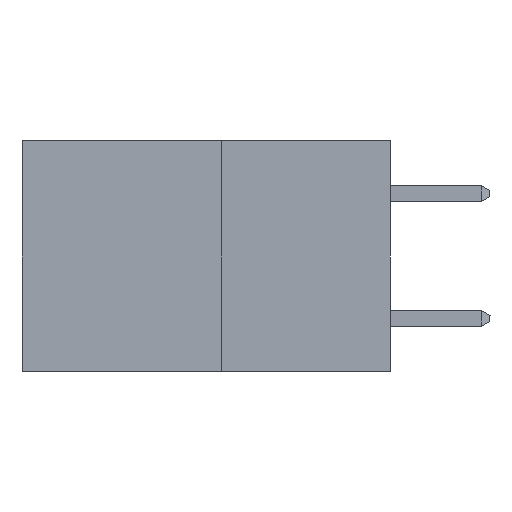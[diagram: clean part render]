
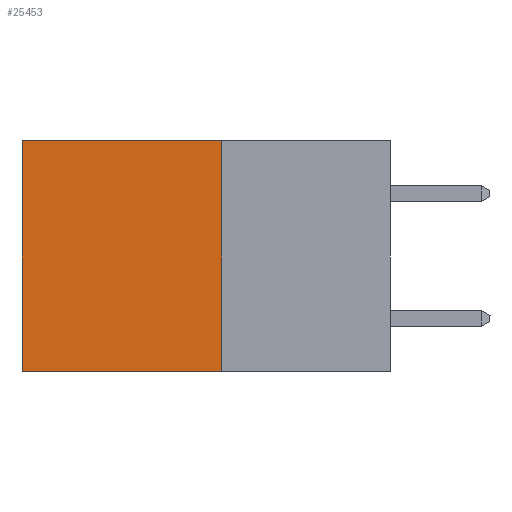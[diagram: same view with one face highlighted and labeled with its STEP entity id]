
A CAD part, left-side view. The second image highlights one B-rep face of the part: STEP entity #25453.
In plain terms, the highlighted planar face has unit normal (-1, 0, 0).
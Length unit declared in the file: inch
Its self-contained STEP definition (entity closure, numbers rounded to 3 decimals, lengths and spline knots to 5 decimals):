
#1934 = VERTEX_POINT ( 'NONE', #5317 ) ;
#2695 = DIRECTION ( 'NONE',  ( 0., 0., -1. ) ) ;
#4121 = EDGE_CURVE ( 'NONE', #22747, #12051, #9934, .T. ) ;
#4200 = ORIENTED_EDGE ( 'NONE', *, *, #4121, .T. ) ;
#5317 = CARTESIAN_POINT ( 'NONE',  ( 0.277, 0.27, 0. ) ) ;
#5670 = ORIENTED_EDGE ( 'NONE', *, *, #5870, .F. ) ;
#5870 = EDGE_CURVE ( 'NONE', #1934, #24438, #7227, .T. ) ;
#6961 = ORIENTED_EDGE ( 'NONE', *, *, #7106, .T. ) ;
#7106 = EDGE_CURVE ( 'NONE', #1934, #22747, #26792, .T. ) ;
#7227 = LINE ( 'NONE', #19819, #18918 ) ;
#7507 = CARTESIAN_POINT ( 'NONE',  ( 0.277, 0.27, -0.37 ) ) ;
#9934 = LINE ( 'NONE', #25748, #21575 ) ;
#10127 = CARTESIAN_POINT ( 'NONE',  ( 0.277, 0.59, -0.37 ) ) ;
#12051 = VERTEX_POINT ( 'NONE', #10127 ) ;
#12527 = EDGE_CURVE ( 'NONE', #24438, #12051, #24372, .T. ) ;
#14469 = PLANE ( 'NONE',  #19640 ) ;
#15068 = FACE_OUTER_BOUND ( 'NONE', #20076, .T. ) ;
#16757 = DIRECTION ( 'NONE',  ( 1., 0., 0. ) ) ;
#16781 = VECTOR ( 'NONE', #23798, 39.37008 ) ;
#18918 = VECTOR ( 'NONE', #29790, 39.37008 ) ;
#19404 = CARTESIAN_POINT ( 'NONE',  ( 0.277, 0.27, -0.37 ) ) ;
#19640 = AXIS2_PLACEMENT_3D ( 'NONE', #23631, #16757, #2695 ) ;
#19819 = CARTESIAN_POINT ( 'NONE',  ( 0.277, 0.27, -0.37 ) ) ;
#20076 = EDGE_LOOP ( 'NONE', ( #4200, #27887, #5670, #6961 ) ) ;
#20478 = CARTESIAN_POINT ( 'NONE',  ( 0.277, 0.59, 0. ) ) ;
#20780 = DIRECTION ( 'NONE',  ( 0., 1., 0. ) ) ;
#21409 = CARTESIAN_POINT ( 'NONE',  ( 0.277, 0.27, 0. ) ) ;
#21575 = VECTOR ( 'NONE', #24347, 39.37008 ) ;
#22747 = VERTEX_POINT ( 'NONE', #20478 ) ;
#23631 = CARTESIAN_POINT ( 'NONE',  ( 0.277, 0.27, -0.37 ) ) ;
#23798 = DIRECTION ( 'NONE',  ( 0., 1., 0. ) ) ;
#24347 = DIRECTION ( 'NONE',  ( 0., 0., -1. ) ) ;
#24372 = LINE ( 'NONE', #7507, #16781 ) ;
#24438 = VERTEX_POINT ( 'NONE', #19404 ) ;
#25369 = VECTOR ( 'NONE', #20780, 39.37008 ) ;
#25453 = ADVANCED_FACE ( 'NONE', ( #15068 ), #14469, .F. ) ;
#25748 = CARTESIAN_POINT ( 'NONE',  ( 0.277, 0.59, -0.37 ) ) ;
#26792 = LINE ( 'NONE', #21409, #25369 ) ;
#27887 = ORIENTED_EDGE ( 'NONE', *, *, #12527, .F. ) ;
#29790 = DIRECTION ( 'NONE',  ( 0., 0., -1. ) ) ;
